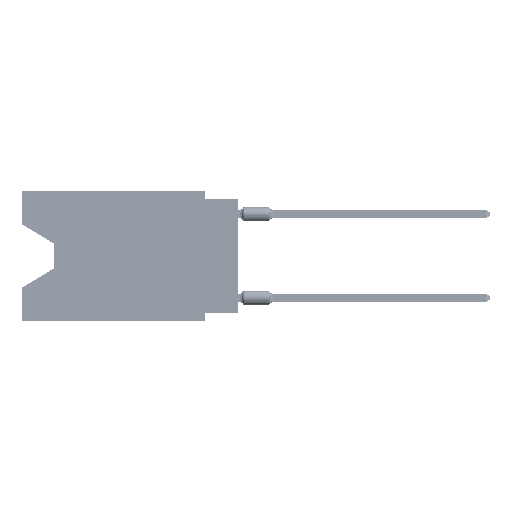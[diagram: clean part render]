
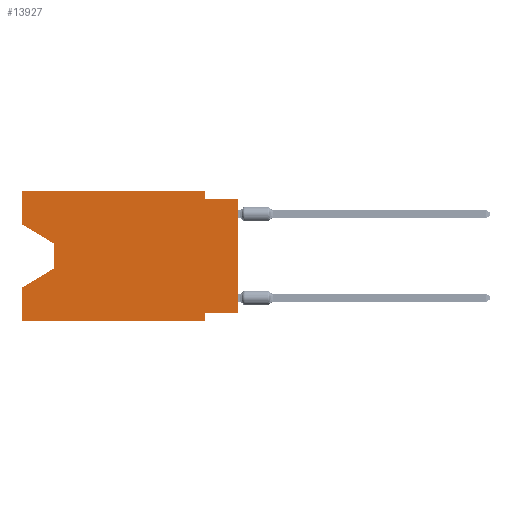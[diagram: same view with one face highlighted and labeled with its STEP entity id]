
A CAD part, left-side view. The second image highlights one B-rep face of the part: STEP entity #13927.
In plain terms, the highlighted planar face has unit normal (-1, 0, 0).
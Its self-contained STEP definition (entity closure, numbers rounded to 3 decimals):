
#819 = CARTESIAN_POINT ( 'NONE',  ( 0., 16.383, -7.36 ) ) ;
#2204 = VERTEX_POINT ( 'NONE', #33751 ) ;
#2352 = DIRECTION ( 'NONE',  ( 0., 0., 1. ) ) ;
#3109 = LINE ( 'NONE', #61983, #22682 ) ;
#8075 = VECTOR ( 'NONE', #28294, 1000. ) ;
#9613 = LINE ( 'NONE', #14638, #24996 ) ;
#9689 = CARTESIAN_POINT ( 'NONE',  ( 0., 0., -0.635 ) ) ;
#10085 = DIRECTION ( 'NONE',  ( 0., 0.855, -0.519 ) ) ;
#10404 = DIRECTION ( 'NONE',  ( 0., 0., -1. ) ) ;
#13557 = EDGE_LOOP ( 'NONE', ( #29281, #30429, #51202, #23980, #42552, #73723, #51387, #28858, #20560, #74079, #43837, #42818 ) ) ;
#13927 = ADVANCED_FACE ( 'NONE', ( #45147 ), #75879, .F. ) ;
#14418 = EDGE_CURVE ( 'NONE', #32254, #31205, #56647, .T. ) ;
#14638 = CARTESIAN_POINT ( 'NONE',  ( 0., 16.383, -9.906 ) ) ;
#14899 = DIRECTION ( 'NONE',  ( 0., -0.855, -0.519 ) ) ;
#15861 = CARTESIAN_POINT ( 'NONE',  ( 0., 13.97, -5.893 ) ) ;
#16019 = LINE ( 'NONE', #39869, #55771 ) ;
#16178 = LINE ( 'NONE', #39663, #66872 ) ;
#19706 = EDGE_CURVE ( 'NONE', #31205, #75477, #68858, .T. ) ;
#20560 = ORIENTED_EDGE ( 'NONE', *, *, #31493, .F. ) ;
#22682 = VECTOR ( 'NONE', #2352, 1000. ) ;
#23112 = CARTESIAN_POINT ( 'NONE',  ( 0., 16.383, -9.906 ) ) ;
#23176 = DIRECTION ( 'NONE',  ( 0., 0., -1. ) ) ;
#23980 = ORIENTED_EDGE ( 'NONE', *, *, #75377, .F. ) ;
#24335 = CARTESIAN_POINT ( 'NONE',  ( 0., 13.97, -4.013 ) ) ;
#24996 = VECTOR ( 'NONE', #67721, 1000. ) ;
#25060 = VECTOR ( 'NONE', #57319, 1000. ) ;
#25799 = VECTOR ( 'NONE', #40076, 1000. ) ;
#27392 = CARTESIAN_POINT ( 'NONE',  ( 0., 16.383, 0. ) ) ;
#27808 = CARTESIAN_POINT ( 'NONE',  ( 0., 16.383, 0. ) ) ;
#27910 = CARTESIAN_POINT ( 'NONE',  ( 0., 13.97, -5.893 ) ) ;
#27934 = CARTESIAN_POINT ( 'NONE',  ( 0., 0., -9.271 ) ) ;
#28095 = VERTEX_POINT ( 'NONE', #52496 ) ;
#28144 = DIRECTION ( 'NONE',  ( 0., 0., 1. ) ) ;
#28294 = DIRECTION ( 'NONE',  ( 0., 1., 0. ) ) ;
#28365 = VECTOR ( 'NONE', #28144, 1000. ) ;
#28858 = ORIENTED_EDGE ( 'NONE', *, *, #49792, .T. ) ;
#29281 = ORIENTED_EDGE ( 'NONE', *, *, #53890, .T. ) ;
#30429 = ORIENTED_EDGE ( 'NONE', *, *, #47552, .T. ) ;
#31205 = VERTEX_POINT ( 'NONE', #71678 ) ;
#31493 = EDGE_CURVE ( 'NONE', #55334, #45605, #39699, .T. ) ;
#32254 = VERTEX_POINT ( 'NONE', #45676 ) ;
#32713 = EDGE_CURVE ( 'NONE', #59198, #32799, #45122, .T. ) ;
#32799 = VERTEX_POINT ( 'NONE', #819 ) ;
#33751 = CARTESIAN_POINT ( 'NONE',  ( 0., 2.54, -9.906 ) ) ;
#35066 = VECTOR ( 'NONE', #57329, 1000. ) ;
#37097 = EDGE_CURVE ( 'NONE', #46838, #2204, #9613, .T. ) ;
#38129 = EDGE_CURVE ( 'NONE', #75477, #55334, #16178, .T. ) ;
#38503 = CARTESIAN_POINT ( 'NONE',  ( 0., 16.383, 0. ) ) ;
#39663 = CARTESIAN_POINT ( 'NONE',  ( 0., 2.54, 0. ) ) ;
#39699 = LINE ( 'NONE', #9689, #25799 ) ;
#39869 = CARTESIAN_POINT ( 'NONE',  ( 0., 0., 0. ) ) ;
#40030 = CARTESIAN_POINT ( 'NONE',  ( 0., 2.54, 0. ) ) ;
#40076 = DIRECTION ( 'NONE',  ( 0., -1., 0. ) ) ;
#40121 = DIRECTION ( 'NONE',  ( 1., 0., 0. ) ) ;
#40607 = CARTESIAN_POINT ( 'NONE',  ( 0., 0., -0.635 ) ) ;
#40768 = CARTESIAN_POINT ( 'NONE',  ( 0., 2.54, -9.906 ) ) ;
#41085 = VERTEX_POINT ( 'NONE', #60406 ) ;
#42308 = VERTEX_POINT ( 'NONE', #24335 ) ;
#42552 = ORIENTED_EDGE ( 'NONE', *, *, #37097, .T. ) ;
#42818 = ORIENTED_EDGE ( 'NONE', *, *, #14418, .F. ) ;
#43837 = ORIENTED_EDGE ( 'NONE', *, *, #19706, .F. ) ;
#45122 = LINE ( 'NONE', #15861, #50515 ) ;
#45147 = FACE_OUTER_BOUND ( 'NONE', #13557, .T. ) ;
#45605 = VERTEX_POINT ( 'NONE', #40607 ) ;
#45676 = CARTESIAN_POINT ( 'NONE',  ( 0., 16.383, -2.546 ) ) ;
#46838 = VERTEX_POINT ( 'NONE', #23112 ) ;
#47552 = EDGE_CURVE ( 'NONE', #42308, #59198, #48022, .T. ) ;
#48022 = LINE ( 'NONE', #73392, #65314 ) ;
#49792 = EDGE_CURVE ( 'NONE', #28095, #45605, #16019, .T. ) ;
#50515 = VECTOR ( 'NONE', #10085, 1000. ) ;
#51202 = ORIENTED_EDGE ( 'NONE', *, *, #32713, .T. ) ;
#51387 = ORIENTED_EDGE ( 'NONE', *, *, #67285, .F. ) ;
#51414 = DIRECTION ( 'NONE',  ( 0., 0., 1. ) ) ;
#51424 = DIRECTION ( 'NONE',  ( 0., 0., -1. ) ) ;
#52496 = CARTESIAN_POINT ( 'NONE',  ( 0., 0., -9.271 ) ) ;
#53890 = EDGE_CURVE ( 'NONE', #32254, #42308, #62205, .T. ) ;
#55334 = VERTEX_POINT ( 'NONE', #56432 ) ;
#55771 = VECTOR ( 'NONE', #51414, 1000. ) ;
#56432 = CARTESIAN_POINT ( 'NONE',  ( 0., 2.54, -0.635 ) ) ;
#56647 = LINE ( 'NONE', #27392, #28365 ) ;
#57319 = DIRECTION ( 'NONE',  ( 0., -1., 0. ) ) ;
#57329 = DIRECTION ( 'NONE',  ( 0., 0., -1. ) ) ;
#57912 = LINE ( 'NONE', #27934, #8075 ) ;
#59198 = VERTEX_POINT ( 'NONE', #27910 ) ;
#60406 = CARTESIAN_POINT ( 'NONE',  ( 0., 2.54, -9.271 ) ) ;
#61983 = CARTESIAN_POINT ( 'NONE',  ( 0., 16.383, 0. ) ) ;
#62205 = LINE ( 'NONE', #67607, #68257 ) ;
#65314 = VECTOR ( 'NONE', #51424, 1000. ) ;
#66507 = AXIS2_PLACEMENT_3D ( 'NONE', #27808, #40121, #23176 ) ;
#66872 = VECTOR ( 'NONE', #10404, 1000. ) ;
#67285 = EDGE_CURVE ( 'NONE', #28095, #41085, #57912, .T. ) ;
#67607 = CARTESIAN_POINT ( 'NONE',  ( 0., 16.383, -2.546 ) ) ;
#67721 = DIRECTION ( 'NONE',  ( 0., -1., 0. ) ) ;
#68257 = VECTOR ( 'NONE', #14899, 1000. ) ;
#68495 = LINE ( 'NONE', #40768, #35066 ) ;
#68858 = LINE ( 'NONE', #38503, #25060 ) ;
#71678 = CARTESIAN_POINT ( 'NONE',  ( 0., 16.383, 0. ) ) ;
#73392 = CARTESIAN_POINT ( 'NONE',  ( 0., 13.97, -4.013 ) ) ;
#73723 = ORIENTED_EDGE ( 'NONE', *, *, #75653, .F. ) ;
#74079 = ORIENTED_EDGE ( 'NONE', *, *, #38129, .F. ) ;
#75377 = EDGE_CURVE ( 'NONE', #46838, #32799, #3109, .T. ) ;
#75477 = VERTEX_POINT ( 'NONE', #40030 ) ;
#75653 = EDGE_CURVE ( 'NONE', #41085, #2204, #68495, .T. ) ;
#75879 = PLANE ( 'NONE',  #66507 ) ;
